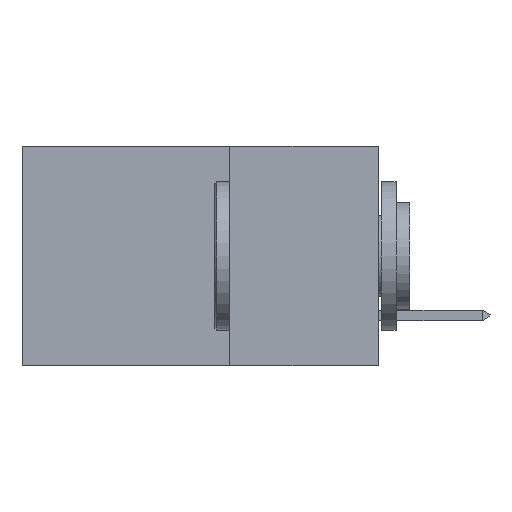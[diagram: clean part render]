
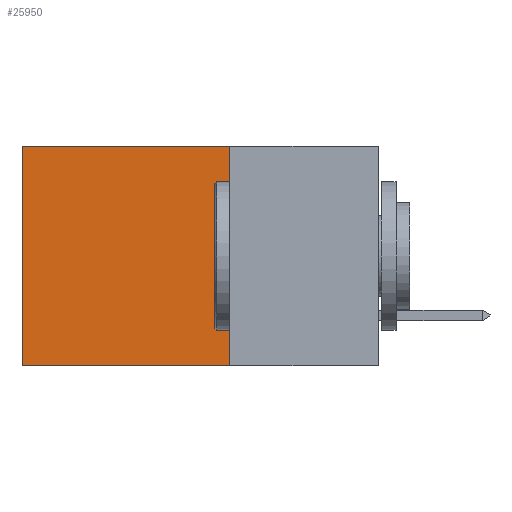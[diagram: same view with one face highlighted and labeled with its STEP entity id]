
A CAD part, left-side view. The second image highlights one B-rep face of the part: STEP entity #25950.
In plain terms, the highlighted planar face has unit normal (-1, 0, 0).
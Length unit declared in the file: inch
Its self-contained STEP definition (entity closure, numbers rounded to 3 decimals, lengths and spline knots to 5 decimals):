
#430 = EDGE_CURVE ( 'NONE', #25746, #25618, #8254, .T. ) ;
#1525 = VECTOR ( 'NONE', #24667, 39.37008 ) ;
#1565 = EDGE_CURVE ( 'NONE', #13625, #25618, #4830, .T. ) ;
#2049 = DIRECTION ( 'NONE',  ( 0., 0., -1. ) ) ;
#2362 = ORIENTED_EDGE ( 'NONE', *, *, #1565, .F. ) ;
#3449 = CARTESIAN_POINT ( 'NONE',  ( 0.298, 0.25, 0. ) ) ;
#3461 = DIRECTION ( 'NONE',  ( 0., 0., -1. ) ) ;
#3533 = PLANE ( 'NONE',  #13610 ) ;
#4608 = VECTOR ( 'NONE', #2049, 39.37008 ) ;
#4765 = CARTESIAN_POINT ( 'NONE',  ( 0.298, 0.25, 0. ) ) ;
#4830 = LINE ( 'NONE', #22470, #1525 ) ;
#4869 = FACE_OUTER_BOUND ( 'NONE', #24053, .T. ) ;
#5612 = CARTESIAN_POINT ( 'NONE',  ( 0.298, 0.6, 0. ) ) ;
#7250 = VECTOR ( 'NONE', #3461, 39.37008 ) ;
#8254 = LINE ( 'NONE', #5612, #7250 ) ;
#8621 = LINE ( 'NONE', #16990, #4608 ) ;
#9565 = CARTESIAN_POINT ( 'NONE',  ( 0.298, 0.25, -0.37 ) ) ;
#9932 = CARTESIAN_POINT ( 'NONE',  ( 0.298, 0.25, 0. ) ) ;
#11054 = ORIENTED_EDGE ( 'NONE', *, *, #13975, .T. ) ;
#13087 = CARTESIAN_POINT ( 'NONE',  ( 0.298, 0.6, -0.37 ) ) ;
#13610 = AXIS2_PLACEMENT_3D ( 'NONE', #3449, #22736, #22548 ) ;
#13625 = VERTEX_POINT ( 'NONE', #9565 ) ;
#13719 = ORIENTED_EDGE ( 'NONE', *, *, #21084, .F. ) ;
#13975 = EDGE_CURVE ( 'NONE', #25642, #25746, #24973, .T. ) ;
#16990 = CARTESIAN_POINT ( 'NONE',  ( 0.298, 0.25, 0. ) ) ;
#19642 = VECTOR ( 'NONE', #24950, 39.37008 ) ;
#21084 = EDGE_CURVE ( 'NONE', #25642, #13625, #8621, .T. ) ;
#22470 = CARTESIAN_POINT ( 'NONE',  ( 0.298, 0.25, -0.37 ) ) ;
#22548 = DIRECTION ( 'NONE',  ( 0., 0., -1. ) ) ;
#22736 = DIRECTION ( 'NONE',  ( 1., 0., 0. ) ) ;
#23930 = CARTESIAN_POINT ( 'NONE',  ( 0.298, 0.6, 0. ) ) ;
#24053 = EDGE_LOOP ( 'NONE', ( #24211, #2362, #13719, #11054 ) ) ;
#24211 = ORIENTED_EDGE ( 'NONE', *, *, #430, .T. ) ;
#24667 = DIRECTION ( 'NONE',  ( 0., 1., 0. ) ) ;
#24950 = DIRECTION ( 'NONE',  ( 0., 1., 0. ) ) ;
#24973 = LINE ( 'NONE', #9932, #19642 ) ;
#25618 = VERTEX_POINT ( 'NONE', #13087 ) ;
#25642 = VERTEX_POINT ( 'NONE', #4765 ) ;
#25746 = VERTEX_POINT ( 'NONE', #23930 ) ;
#25950 = ADVANCED_FACE ( 'NONE', ( #4869 ), #3533, .F. ) ;
